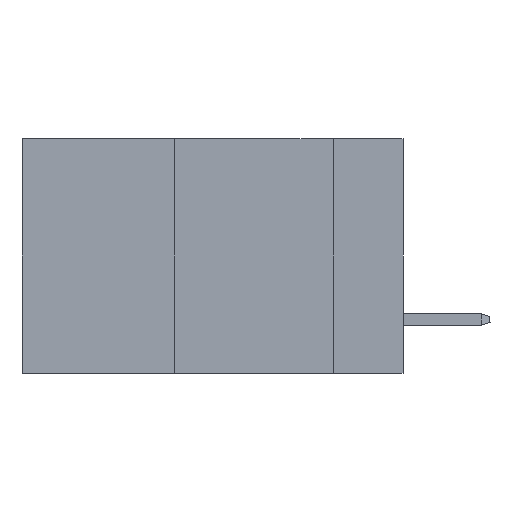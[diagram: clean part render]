
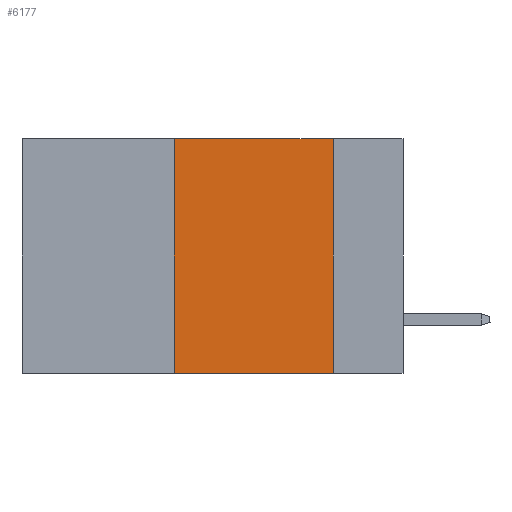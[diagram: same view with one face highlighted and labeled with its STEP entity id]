
A CAD part, left-side view. The second image highlights one B-rep face of the part: STEP entity #6177.
In plain terms, the highlighted planar face has unit normal (-1, 0, 0).
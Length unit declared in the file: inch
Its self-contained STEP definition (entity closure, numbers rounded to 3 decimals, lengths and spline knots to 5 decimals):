
#731 = CARTESIAN_POINT ( 'NONE',  ( 0., 0.11, -0.37 ) ) ;
#818 = CARTESIAN_POINT ( 'NONE',  ( 0., 0.11, 0. ) ) ;
#1665 = LINE ( 'NONE', #31393, #5689 ) ;
#1764 = VERTEX_POINT ( 'NONE', #731 ) ;
#2248 = VERTEX_POINT ( 'NONE', #34479 ) ;
#2915 = DIRECTION ( 'NONE',  ( 0., 0., 1. ) ) ;
#4229 = EDGE_CURVE ( 'NONE', #4878, #1764, #39404, .T. ) ;
#4845 = LINE ( 'NONE', #14712, #27718 ) ;
#4878 = VERTEX_POINT ( 'NONE', #818 ) ;
#5689 = VECTOR ( 'NONE', #41005, 39.37008 ) ;
#6106 = LINE ( 'NONE', #33421, #39132 ) ;
#6177 = ADVANCED_FACE ( 'NONE', ( #39774 ), #36569, .F. ) ;
#7818 = EDGE_CURVE ( 'NONE', #35530, #2248, #6106, .T. ) ;
#7876 = CARTESIAN_POINT ( 'NONE',  ( 0., 0.6, 0. ) ) ;
#8854 = EDGE_LOOP ( 'NONE', ( #40295, #18051, #9095, #9843 ) ) ;
#9095 = ORIENTED_EDGE ( 'NONE', *, *, #7818, .F. ) ;
#9843 = ORIENTED_EDGE ( 'NONE', *, *, #38502, .T. ) ;
#14712 = CARTESIAN_POINT ( 'NONE',  ( 0., 0.6, 0. ) ) ;
#18051 = ORIENTED_EDGE ( 'NONE', *, *, #41714, .F. ) ;
#20307 = DIRECTION ( 'NONE',  ( 0., 0., -1. ) ) ;
#20900 = VECTOR ( 'NONE', #38978, 39.37008 ) ;
#21317 = DIRECTION ( 'NONE',  ( 0., -1., 0. ) ) ;
#27718 = VECTOR ( 'NONE', #21317, 39.37008 ) ;
#31393 = CARTESIAN_POINT ( 'NONE',  ( 0., 0.6, -0.37 ) ) ;
#32178 = AXIS2_PLACEMENT_3D ( 'NONE', #7876, #33562, #20307 ) ;
#33421 = CARTESIAN_POINT ( 'NONE',  ( 0., 0.36, 0. ) ) ;
#33562 = DIRECTION ( 'NONE',  ( 1., 0., 0. ) ) ;
#34479 = CARTESIAN_POINT ( 'NONE',  ( 0., 0.36, 0. ) ) ;
#35530 = VERTEX_POINT ( 'NONE', #38275 ) ;
#36569 = PLANE ( 'NONE',  #32178 ) ;
#38275 = CARTESIAN_POINT ( 'NONE',  ( 0., 0.36, -0.37 ) ) ;
#38502 = EDGE_CURVE ( 'NONE', #35530, #1764, #1665, .T. ) ;
#38978 = DIRECTION ( 'NONE',  ( 0., 0., -1. ) ) ;
#39132 = VECTOR ( 'NONE', #2915, 39.37008 ) ;
#39404 = LINE ( 'NONE', #41979, #20900 ) ;
#39774 = FACE_OUTER_BOUND ( 'NONE', #8854, .T. ) ;
#40295 = ORIENTED_EDGE ( 'NONE', *, *, #4229, .F. ) ;
#41005 = DIRECTION ( 'NONE',  ( 0., -1., 0. ) ) ;
#41714 = EDGE_CURVE ( 'NONE', #2248, #4878, #4845, .T. ) ;
#41979 = CARTESIAN_POINT ( 'NONE',  ( 0., 0.11, 0. ) ) ;
